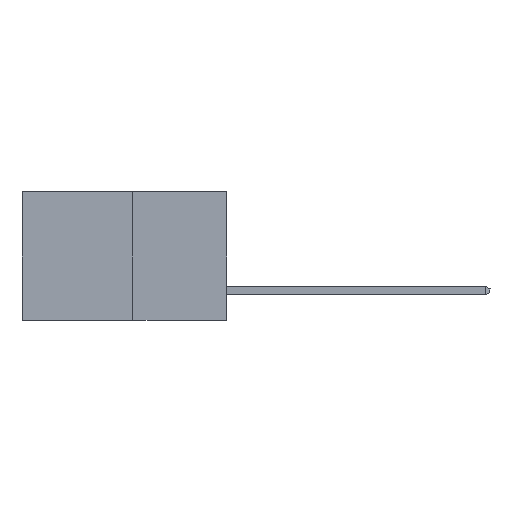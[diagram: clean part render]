
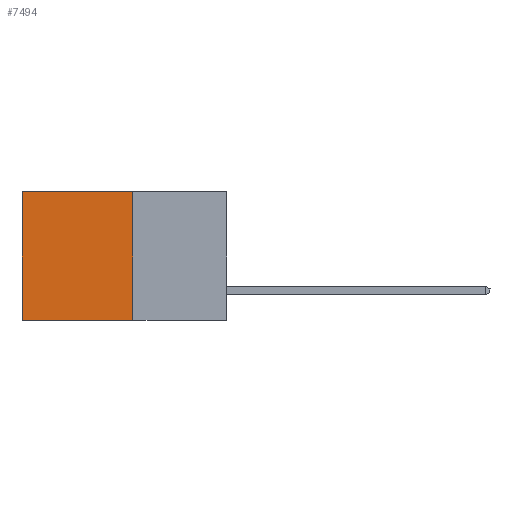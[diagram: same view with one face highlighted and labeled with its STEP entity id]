
A CAD part, left-side view. The second image highlights one B-rep face of the part: STEP entity #7494.
In plain terms, the highlighted planar face has unit normal (-1, 0, 0).
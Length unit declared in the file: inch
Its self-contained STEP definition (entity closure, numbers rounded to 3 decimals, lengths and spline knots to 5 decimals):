
#163 = DIRECTION ( 'NONE',  ( 0., 0., -1. ) ) ;
#170 = CARTESIAN_POINT ( 'NONE',  ( 0.277, 0.27, -0.37 ) ) ;
#248 = CARTESIAN_POINT ( 'NONE',  ( 0.277, 0.27, -0.37 ) ) ;
#995 = ORIENTED_EDGE ( 'NONE', *, *, #6949, .T. ) ;
#1378 = LINE ( 'NONE', #248, #13285 ) ;
#1775 = DIRECTION ( 'NONE',  ( 0., 1., 0. ) ) ;
#1938 = CARTESIAN_POINT ( 'NONE',  ( 0.277, 0.27, 0. ) ) ;
#2949 = VECTOR ( 'NONE', #11052, 39.37008 ) ;
#3415 = VECTOR ( 'NONE', #4391, 39.37008 ) ;
#3773 = VERTEX_POINT ( 'NONE', #10995 ) ;
#3808 = AXIS2_PLACEMENT_3D ( 'NONE', #170, #6574, #14571 ) ;
#4391 = DIRECTION ( 'NONE',  ( 0., 1., 0. ) ) ;
#6129 = LINE ( 'NONE', #13286, #2949 ) ;
#6574 = DIRECTION ( 'NONE',  ( 1., 0., 0. ) ) ;
#6581 = EDGE_CURVE ( 'NONE', #8781, #3773, #1378, .T. ) ;
#6949 = EDGE_CURVE ( 'NONE', #8781, #15268, #13966, .T. ) ;
#7400 = VERTEX_POINT ( 'NONE', #14334 ) ;
#7494 = ADVANCED_FACE ( 'NONE', ( #11121 ), #13476, .F. ) ;
#7917 = VECTOR ( 'NONE', #1775, 39.37008 ) ;
#8781 = VERTEX_POINT ( 'NONE', #1938 ) ;
#9629 = EDGE_LOOP ( 'NONE', ( #11400, #14703, #10171, #995 ) ) ;
#10117 = CARTESIAN_POINT ( 'NONE',  ( 0.277, 0.59, 0. ) ) ;
#10143 = EDGE_CURVE ( 'NONE', #3773, #7400, #12779, .T. ) ;
#10171 = ORIENTED_EDGE ( 'NONE', *, *, #6581, .F. ) ;
#10995 = CARTESIAN_POINT ( 'NONE',  ( 0.277, 0.27, -0.37 ) ) ;
#11052 = DIRECTION ( 'NONE',  ( 0., 0., -1. ) ) ;
#11121 = FACE_OUTER_BOUND ( 'NONE', #9629, .T. ) ;
#11400 = ORIENTED_EDGE ( 'NONE', *, *, #14399, .T. ) ;
#12779 = LINE ( 'NONE', #14751, #3415 ) ;
#13285 = VECTOR ( 'NONE', #163, 39.37008 ) ;
#13286 = CARTESIAN_POINT ( 'NONE',  ( 0.277, 0.59, -0.37 ) ) ;
#13476 = PLANE ( 'NONE',  #3808 ) ;
#13966 = LINE ( 'NONE', #14637, #7917 ) ;
#14334 = CARTESIAN_POINT ( 'NONE',  ( 0.277, 0.59, -0.37 ) ) ;
#14399 = EDGE_CURVE ( 'NONE', #15268, #7400, #6129, .T. ) ;
#14571 = DIRECTION ( 'NONE',  ( 0., 0., -1. ) ) ;
#14637 = CARTESIAN_POINT ( 'NONE',  ( 0.277, 0.27, 0. ) ) ;
#14703 = ORIENTED_EDGE ( 'NONE', *, *, #10143, .F. ) ;
#14751 = CARTESIAN_POINT ( 'NONE',  ( 0.277, 0.27, -0.37 ) ) ;
#15268 = VERTEX_POINT ( 'NONE', #10117 ) ;
